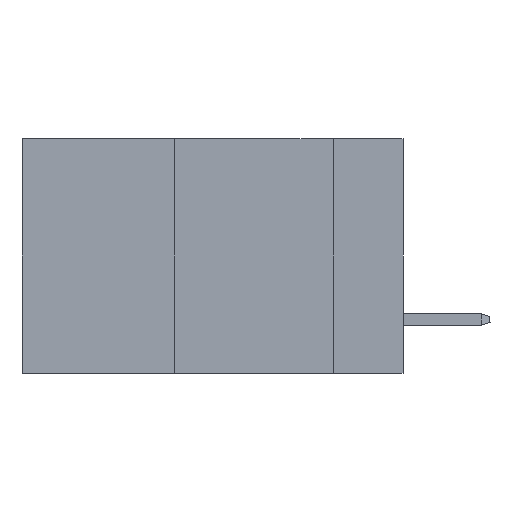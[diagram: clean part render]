
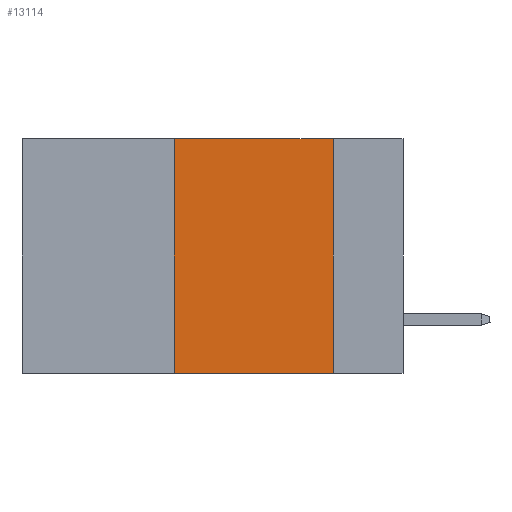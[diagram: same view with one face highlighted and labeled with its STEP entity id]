
A CAD part, left-side view. The second image highlights one B-rep face of the part: STEP entity #13114.
In plain terms, the highlighted planar face has unit normal (-1, 0, 0).
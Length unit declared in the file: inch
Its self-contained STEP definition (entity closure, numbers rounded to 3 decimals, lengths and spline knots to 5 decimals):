
#275 = ORIENTED_EDGE ( 'NONE', *, *, #11751, .F. ) ;
#1464 = CARTESIAN_POINT ( 'NONE',  ( 0., 0.6, -0.37 ) ) ;
#1679 = DIRECTION ( 'NONE',  ( 0., -1., 0. ) ) ;
#1968 = VERTEX_POINT ( 'NONE', #5080 ) ;
#3243 = DIRECTION ( 'NONE',  ( 1., 0., 0. ) ) ;
#4004 = VECTOR ( 'NONE', #21801, 39.37008 ) ;
#5080 = CARTESIAN_POINT ( 'NONE',  ( 0., 0.36, -0.37 ) ) ;
#5435 = CARTESIAN_POINT ( 'NONE',  ( 0., 0.6, 0. ) ) ;
#5892 = DIRECTION ( 'NONE',  ( 0., 0., -1. ) ) ;
#6085 = VECTOR ( 'NONE', #5892, 39.37008 ) ;
#6169 = LINE ( 'NONE', #14818, #4004 ) ;
#6362 = VERTEX_POINT ( 'NONE', #8252 ) ;
#7275 = ORIENTED_EDGE ( 'NONE', *, *, #11124, .F. ) ;
#7357 = AXIS2_PLACEMENT_3D ( 'NONE', #18548, #3243, #18866 ) ;
#7840 = CARTESIAN_POINT ( 'NONE',  ( 0., 0.11, 0. ) ) ;
#7867 = ORIENTED_EDGE ( 'NONE', *, *, #11044, .T. ) ;
#8252 = CARTESIAN_POINT ( 'NONE',  ( 0., 0.36, 0. ) ) ;
#8258 = PLANE ( 'NONE',  #7357 ) ;
#8702 = VECTOR ( 'NONE', #1679, 39.37008 ) ;
#9445 = VERTEX_POINT ( 'NONE', #16635 ) ;
#9890 = EDGE_CURVE ( 'NONE', #10602, #9445, #16260, .T. ) ;
#10602 = VERTEX_POINT ( 'NONE', #11851 ) ;
#11044 = EDGE_CURVE ( 'NONE', #1968, #9445, #13522, .T. ) ;
#11124 = EDGE_CURVE ( 'NONE', #6362, #10602, #21272, .T. ) ;
#11751 = EDGE_CURVE ( 'NONE', #1968, #6362, #6169, .T. ) ;
#11851 = CARTESIAN_POINT ( 'NONE',  ( 0., 0.11, 0. ) ) ;
#12481 = DIRECTION ( 'NONE',  ( 0., -1., 0. ) ) ;
#13114 = ADVANCED_FACE ( 'NONE', ( #18648 ), #8258, .F. ) ;
#13522 = LINE ( 'NONE', #1464, #8702 ) ;
#14818 = CARTESIAN_POINT ( 'NONE',  ( 0., 0.36, 0. ) ) ;
#16260 = LINE ( 'NONE', #7840, #6085 ) ;
#16635 = CARTESIAN_POINT ( 'NONE',  ( 0., 0.11, -0.37 ) ) ;
#18548 = CARTESIAN_POINT ( 'NONE',  ( 0., 0.6, 0. ) ) ;
#18648 = FACE_OUTER_BOUND ( 'NONE', #22538, .T. ) ;
#18866 = DIRECTION ( 'NONE',  ( 0., 0., -1. ) ) ;
#18905 = VECTOR ( 'NONE', #12481, 39.37008 ) ;
#20278 = ORIENTED_EDGE ( 'NONE', *, *, #9890, .F. ) ;
#21272 = LINE ( 'NONE', #5435, #18905 ) ;
#21801 = DIRECTION ( 'NONE',  ( 0., 0., 1. ) ) ;
#22538 = EDGE_LOOP ( 'NONE', ( #20278, #7275, #275, #7867 ) ) ;
